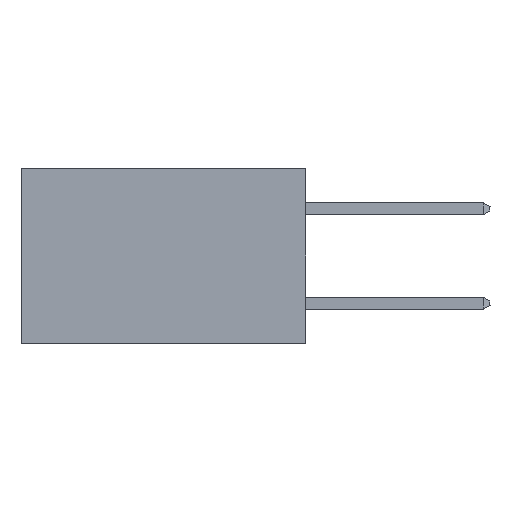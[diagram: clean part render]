
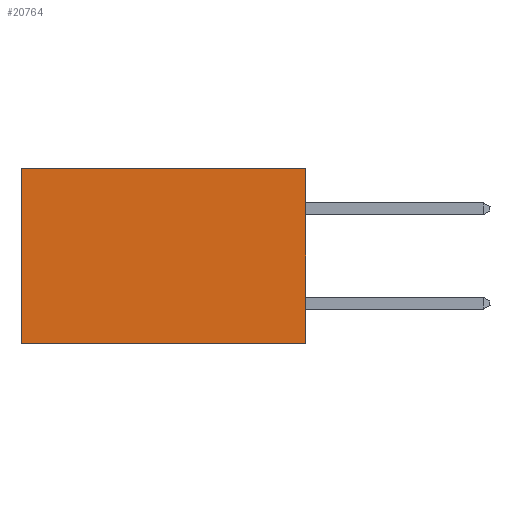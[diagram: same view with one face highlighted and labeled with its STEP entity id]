
A CAD part, left-side view. The second image highlights one B-rep face of the part: STEP entity #20764.
In plain terms, the highlighted planar face has unit normal (-1, 0, 0).
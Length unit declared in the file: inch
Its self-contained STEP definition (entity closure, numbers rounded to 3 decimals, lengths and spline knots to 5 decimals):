
#46 = DIRECTION ( 'NONE',  ( 0., 1., 0. ) ) ;
#714 = ORIENTED_EDGE ( 'NONE', *, *, #20765, .T. ) ;
#1252 = EDGE_CURVE ( 'NONE', #10364, #18875, #21040, .T. ) ;
#2829 = CARTESIAN_POINT ( 'NONE',  ( 0.298, 0.6, 0. ) ) ;
#3064 = DIRECTION ( 'NONE',  ( 0., 0., -1. ) ) ;
#3122 = VERTEX_POINT ( 'NONE', #19007 ) ;
#3344 = VECTOR ( 'NONE', #22540, 39.37008 ) ;
#3786 = AXIS2_PLACEMENT_3D ( 'NONE', #8649, #12298, #3064 ) ;
#5974 = CARTESIAN_POINT ( 'NONE',  ( 0.298, 0., 0. ) ) ;
#6764 = CARTESIAN_POINT ( 'NONE',  ( 0.298, 0.6, 0. ) ) ;
#6798 = DIRECTION ( 'NONE',  ( 0., 1., 0. ) ) ;
#7168 = CARTESIAN_POINT ( 'NONE',  ( 0.298, 0., -0.37 ) ) ;
#7358 = VECTOR ( 'NONE', #6798, 39.37008 ) ;
#8649 = CARTESIAN_POINT ( 'NONE',  ( 0.298, 0., 0. ) ) ;
#10331 = EDGE_CURVE ( 'NONE', #3122, #21282, #16338, .T. ) ;
#10364 = VERTEX_POINT ( 'NONE', #2829 ) ;
#10367 = PLANE ( 'NONE',  #3786 ) ;
#10803 = LINE ( 'NONE', #22420, #19437 ) ;
#11503 = EDGE_LOOP ( 'NONE', ( #21484, #13867, #23807, #714 ) ) ;
#12298 = DIRECTION ( 'NONE',  ( 1., 0., 0. ) ) ;
#12572 = DIRECTION ( 'NONE',  ( 0., 0., -1. ) ) ;
#13854 = CARTESIAN_POINT ( 'NONE',  ( 0.298, 0.6, -0.37 ) ) ;
#13867 = ORIENTED_EDGE ( 'NONE', *, *, #21133, .F. ) ;
#16338 = LINE ( 'NONE', #5974, #3344 ) ;
#17409 = FACE_OUTER_BOUND ( 'NONE', #11503, .T. ) ;
#17818 = CARTESIAN_POINT ( 'NONE',  ( 0.298, 0., 0. ) ) ;
#18875 = VERTEX_POINT ( 'NONE', #13854 ) ;
#19007 = CARTESIAN_POINT ( 'NONE',  ( 0.298, 0., 0. ) ) ;
#19437 = VECTOR ( 'NONE', #46, 39.37008 ) ;
#20764 = ADVANCED_FACE ( 'NONE', ( #17409 ), #10367, .F. ) ;
#20765 = EDGE_CURVE ( 'NONE', #3122, #10364, #22931, .T. ) ;
#21040 = LINE ( 'NONE', #6764, #21333 ) ;
#21133 = EDGE_CURVE ( 'NONE', #21282, #18875, #10803, .T. ) ;
#21282 = VERTEX_POINT ( 'NONE', #7168 ) ;
#21333 = VECTOR ( 'NONE', #12572, 39.37008 ) ;
#21484 = ORIENTED_EDGE ( 'NONE', *, *, #1252, .T. ) ;
#22420 = CARTESIAN_POINT ( 'NONE',  ( 0.298, 0., -0.37 ) ) ;
#22540 = DIRECTION ( 'NONE',  ( 0., 0., -1. ) ) ;
#22931 = LINE ( 'NONE', #17818, #7358 ) ;
#23807 = ORIENTED_EDGE ( 'NONE', *, *, #10331, .F. ) ;
